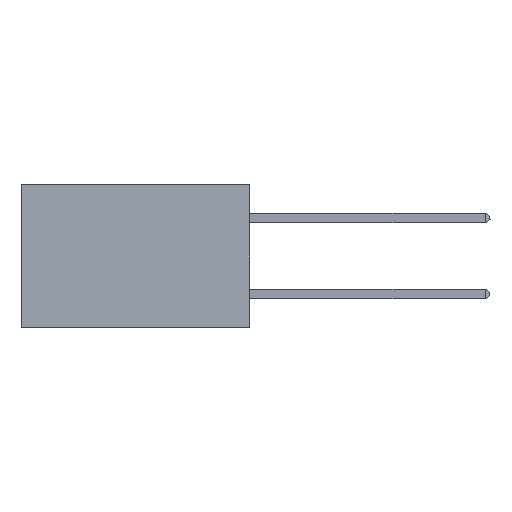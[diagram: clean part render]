
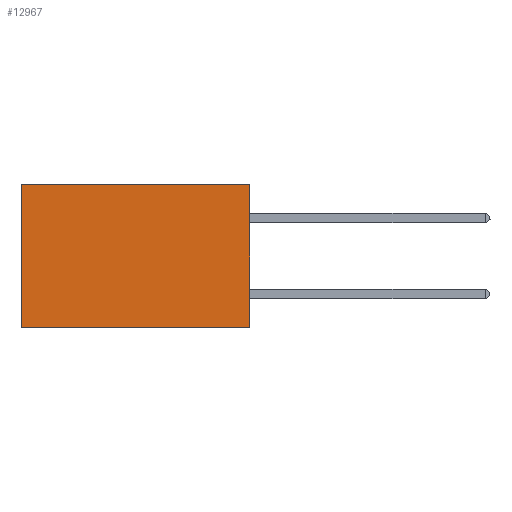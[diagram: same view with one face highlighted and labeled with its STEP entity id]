
A CAD part, left-side view. The second image highlights one B-rep face of the part: STEP entity #12967.
In plain terms, the highlighted planar face has unit normal (-1, 0, 0).
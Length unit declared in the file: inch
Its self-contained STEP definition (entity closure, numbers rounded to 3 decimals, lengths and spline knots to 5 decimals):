
#460 = CARTESIAN_POINT ( 'NONE',  ( 0.2875, 0., -0.375 ) ) ;
#594 = EDGE_CURVE ( 'NONE', #1762, #11343, #10911, .T. ) ;
#1129 = AXIS2_PLACEMENT_3D ( 'NONE', #5924, #13324, #7011 ) ;
#1618 = DIRECTION ( 'NONE',  ( 0., 1., 0. ) ) ;
#1762 = VERTEX_POINT ( 'NONE', #4090 ) ;
#2252 = ORIENTED_EDGE ( 'NONE', *, *, #4028, .F. ) ;
#2334 = LINE ( 'NONE', #4365, #6248 ) ;
#2495 = LINE ( 'NONE', #460, #3567 ) ;
#3372 = EDGE_CURVE ( 'NONE', #11343, #10397, #10122, .T. ) ;
#3567 = VECTOR ( 'NONE', #8747, 39.37008 ) ;
#4028 = EDGE_CURVE ( 'NONE', #8664, #10397, #2334, .T. ) ;
#4090 = CARTESIAN_POINT ( 'NONE',  ( 0.2875, 0., 0. ) ) ;
#4365 = CARTESIAN_POINT ( 'NONE',  ( 0.2875, 0., -0.375 ) ) ;
#4801 = CARTESIAN_POINT ( 'NONE',  ( 0.2875, 0., 0. ) ) ;
#5924 = CARTESIAN_POINT ( 'NONE',  ( 0.2875, 0., -0.375 ) ) ;
#6248 = VECTOR ( 'NONE', #6627, 39.37008 ) ;
#6627 = DIRECTION ( 'NONE',  ( 0., 1., 0. ) ) ;
#6726 = CARTESIAN_POINT ( 'NONE',  ( 0.2875, 0.6, 0. ) ) ;
#7003 = CARTESIAN_POINT ( 'NONE',  ( 0.2875, 0.6, -0.375 ) ) ;
#7011 = DIRECTION ( 'NONE',  ( 0., 0., -1. ) ) ;
#7621 = VECTOR ( 'NONE', #12422, 39.37008 ) ;
#8189 = CARTESIAN_POINT ( 'NONE',  ( 0.2875, 0., -0.375 ) ) ;
#8457 = VECTOR ( 'NONE', #1618, 39.37008 ) ;
#8664 = VERTEX_POINT ( 'NONE', #8189 ) ;
#8747 = DIRECTION ( 'NONE',  ( 0., 0., -1. ) ) ;
#8927 = ORIENTED_EDGE ( 'NONE', *, *, #594, .T. ) ;
#8942 = ORIENTED_EDGE ( 'NONE', *, *, #3372, .T. ) ;
#8944 = EDGE_LOOP ( 'NONE', ( #8942, #2252, #9139, #8927 ) ) ;
#9139 = ORIENTED_EDGE ( 'NONE', *, *, #10402, .F. ) ;
#9175 = PLANE ( 'NONE',  #1129 ) ;
#9828 = CARTESIAN_POINT ( 'NONE',  ( 0.2875, 0.6, -0.375 ) ) ;
#10122 = LINE ( 'NONE', #7003, #7621 ) ;
#10264 = FACE_OUTER_BOUND ( 'NONE', #8944, .T. ) ;
#10397 = VERTEX_POINT ( 'NONE', #9828 ) ;
#10402 = EDGE_CURVE ( 'NONE', #1762, #8664, #2495, .T. ) ;
#10911 = LINE ( 'NONE', #4801, #8457 ) ;
#11343 = VERTEX_POINT ( 'NONE', #6726 ) ;
#12422 = DIRECTION ( 'NONE',  ( 0., 0., -1. ) ) ;
#12967 = ADVANCED_FACE ( 'NONE', ( #10264 ), #9175, .F. ) ;
#13324 = DIRECTION ( 'NONE',  ( 1., 0., 0. ) ) ;
